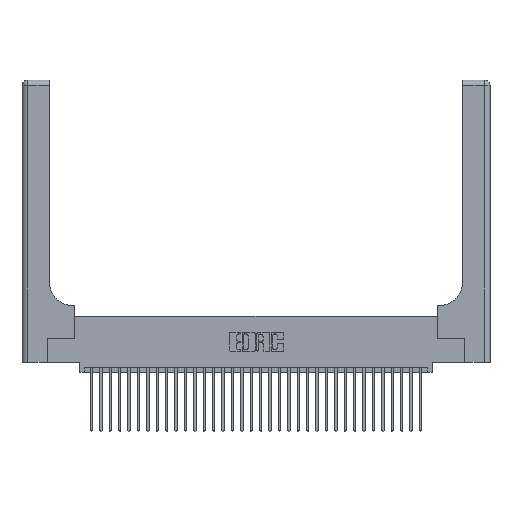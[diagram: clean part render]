
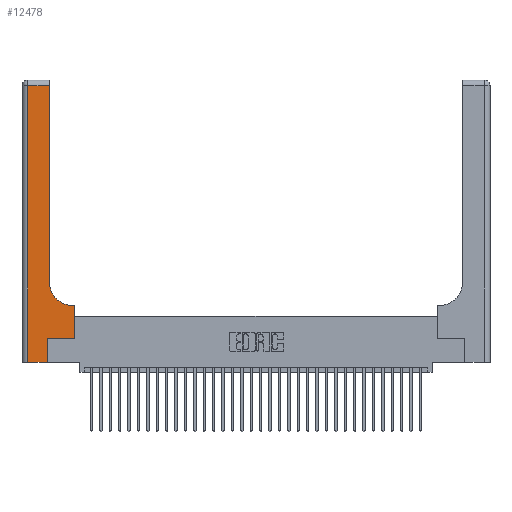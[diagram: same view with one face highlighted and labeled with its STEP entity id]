
A CAD part, top view. The second image highlights one B-rep face of the part: STEP entity #12478.
In plain terms, the highlighted planar face has unit normal (0, 0, 1).
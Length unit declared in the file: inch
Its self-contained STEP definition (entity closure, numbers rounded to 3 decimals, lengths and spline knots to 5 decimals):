
#978 = VERTEX_POINT ( 'NONE', #33614 ) ;
#1079 = VERTEX_POINT ( 'NONE', #23523 ) ;
#1126 = EDGE_CURVE ( 'NONE', #29126, #6556, #30730, .T. ) ;
#1547 = DIRECTION ( 'NONE',  ( 0., -1., 0. ) ) ;
#2019 = CARTESIAN_POINT ( 'NONE',  ( 0., 3., 0.37 ) ) ;
#2145 = DIRECTION ( 'NONE',  ( 0., 0., -1. ) ) ;
#2460 = EDGE_CURVE ( 'NONE', #6471, #14903, #25297, .T. ) ;
#2499 = DIRECTION ( 'NONE',  ( 0., 0., -1. ) ) ;
#3186 = ORIENTED_EDGE ( 'NONE', *, *, #2460, .T. ) ;
#3555 = VECTOR ( 'NONE', #27327, 39.37008 ) ;
#3872 = ORIENTED_EDGE ( 'NONE', *, *, #23093, .T. ) ;
#4370 = CARTESIAN_POINT ( 'NONE',  ( 0.2915, 3., 0.37 ) ) ;
#4413 = LINE ( 'NONE', #16744, #3555 ) ;
#5487 = CARTESIAN_POINT ( 'NONE',  ( 0.269, 0., 0.37 ) ) ;
#6347 = ORIENTED_EDGE ( 'NONE', *, *, #1126, .T. ) ;
#6471 = VERTEX_POINT ( 'NONE', #7690 ) ;
#6556 = VERTEX_POINT ( 'NONE', #29196 ) ;
#6570 = ORIENTED_EDGE ( 'NONE', *, *, #14625, .T. ) ;
#7395 = CARTESIAN_POINT ( 'NONE',  ( 0.269, 0., 0.37 ) ) ;
#7690 = CARTESIAN_POINT ( 'NONE',  ( 0.06, 0., 0.37 ) ) ;
#8786 = DIRECTION ( 'NONE',  ( 0., 1., 0. ) ) ;
#9014 = VERTEX_POINT ( 'NONE', #15691 ) ;
#9389 = DIRECTION ( 'NONE',  ( -1., 0., 0. ) ) ;
#9544 = VECTOR ( 'NONE', #8786, 39.37008 ) ;
#10927 = LINE ( 'NONE', #4370, #31172 ) ;
#11007 = EDGE_CURVE ( 'NONE', #978, #32049, #31454, .T. ) ;
#11944 = CARTESIAN_POINT ( 'NONE',  ( 0.2915, 0.6, 0.37 ) ) ;
#12097 = EDGE_CURVE ( 'NONE', #24245, #978, #4413, .T. ) ;
#12280 = LINE ( 'NONE', #28906, #26351 ) ;
#12478 = ADVANCED_FACE ( 'NONE', ( #28066 ), #31316, .F. ) ;
#12627 = VECTOR ( 'NONE', #9389, 39.37008 ) ;
#13482 = LINE ( 'NONE', #11944, #12627 ) ;
#14625 = EDGE_CURVE ( 'NONE', #32049, #29126, #13482, .T. ) ;
#14903 = VERTEX_POINT ( 'NONE', #5487 ) ;
#15170 = DIRECTION ( 'NONE',  ( 0., 1., 0. ) ) ;
#15691 = CARTESIAN_POINT ( 'NONE',  ( 0.06, 2.94, 0.37 ) ) ;
#15701 = DIRECTION ( 'NONE',  ( -1., 0., 0. ) ) ;
#16280 = CARTESIAN_POINT ( 'NONE',  ( 0., 0., 0.37 ) ) ;
#16744 = CARTESIAN_POINT ( 'NONE',  ( 0.269, 0.25, 0.37 ) ) ;
#17648 = CARTESIAN_POINT ( 'NONE',  ( 0.06, 3., 0.37 ) ) ;
#18598 = CARTESIAN_POINT ( 'NONE',  ( 0.5415, 0.85, 0.37 ) ) ;
#20901 = DIRECTION ( 'NONE',  ( -1., 0., 0. ) ) ;
#21241 = DIRECTION ( 'NONE',  ( 1., 0., 0. ) ) ;
#21514 = VECTOR ( 'NONE', #31338, 39.37008 ) ;
#21930 = EDGE_CURVE ( 'NONE', #1079, #9014, #12280, .T. ) ;
#22958 = AXIS2_PLACEMENT_3D ( 'NONE', #2019, #2145, #20901 ) ;
#23093 = EDGE_CURVE ( 'NONE', #6556, #1079, #10927, .T. ) ;
#23523 = CARTESIAN_POINT ( 'NONE',  ( 0.2915, 2.94, 0.37 ) ) ;
#24245 = VERTEX_POINT ( 'NONE', #33028 ) ;
#24357 = EDGE_CURVE ( 'NONE', #9014, #6471, #31903, .T. ) ;
#25029 = CARTESIAN_POINT ( 'NONE',  ( 0.5415, 0.6, 0.37 ) ) ;
#25297 = LINE ( 'NONE', #16280, #31461 ) ;
#26351 = VECTOR ( 'NONE', #15701, 39.37008 ) ;
#26572 = EDGE_LOOP ( 'NONE', ( #3872, #33116, #27114, #3186, #28500, #34310, #28296, #6570, #6347 ) ) ;
#26760 = DIRECTION ( 'NONE',  ( 1., 0., 0. ) ) ;
#27114 = ORIENTED_EDGE ( 'NONE', *, *, #24357, .T. ) ;
#27327 = DIRECTION ( 'NONE',  ( 1., 0., 0. ) ) ;
#27450 = EDGE_CURVE ( 'NONE', #14903, #24245, #28464, .T. ) ;
#28066 = FACE_OUTER_BOUND ( 'NONE', #26572, .T. ) ;
#28296 = ORIENTED_EDGE ( 'NONE', *, *, #11007, .T. ) ;
#28464 = LINE ( 'NONE', #7395, #21514 ) ;
#28500 = ORIENTED_EDGE ( 'NONE', *, *, #27450, .T. ) ;
#28906 = CARTESIAN_POINT ( 'NONE',  ( 0., 2.94, 0.37 ) ) ;
#29126 = VERTEX_POINT ( 'NONE', #25029 ) ;
#29196 = CARTESIAN_POINT ( 'NONE',  ( 0.2915, 0.85, 0.37 ) ) ;
#30616 = AXIS2_PLACEMENT_3D ( 'NONE', #18598, #2499, #21241 ) ;
#30730 = CIRCLE ( 'NONE', #30616, 0.25 ) ;
#30944 = CARTESIAN_POINT ( 'NONE',  ( 0.5585, 0.6, 0.37 ) ) ;
#31172 = VECTOR ( 'NONE', #15170, 39.37008 ) ;
#31316 = PLANE ( 'NONE',  #22958 ) ;
#31338 = DIRECTION ( 'NONE',  ( 0., 1., 0. ) ) ;
#31454 = LINE ( 'NONE', #32460, #9544 ) ;
#31461 = VECTOR ( 'NONE', #26760, 39.37008 ) ;
#31903 = LINE ( 'NONE', #17648, #32728 ) ;
#32049 = VERTEX_POINT ( 'NONE', #30944 ) ;
#32460 = CARTESIAN_POINT ( 'NONE',  ( 0.5585, 0.25, 0.37 ) ) ;
#32728 = VECTOR ( 'NONE', #1547, 39.37008 ) ;
#33028 = CARTESIAN_POINT ( 'NONE',  ( 0.269, 0.25, 0.37 ) ) ;
#33116 = ORIENTED_EDGE ( 'NONE', *, *, #21930, .T. ) ;
#33614 = CARTESIAN_POINT ( 'NONE',  ( 0.5585, 0.25, 0.37 ) ) ;
#34310 = ORIENTED_EDGE ( 'NONE', *, *, #12097, .T. ) ;
